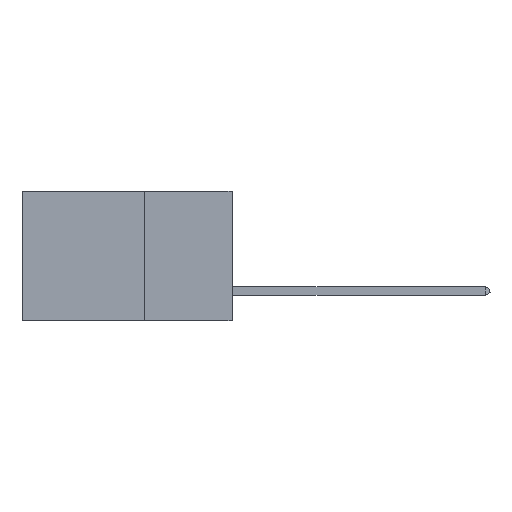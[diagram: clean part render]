
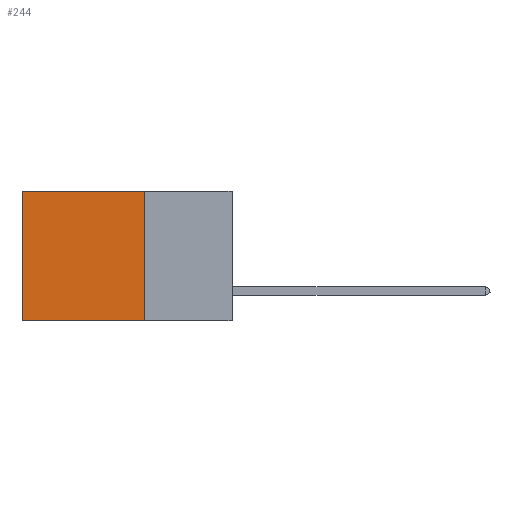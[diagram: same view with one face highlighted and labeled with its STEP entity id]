
A CAD part, left-side view. The second image highlights one B-rep face of the part: STEP entity #244.
In plain terms, the highlighted planar face has unit normal (-1, 0, 0).
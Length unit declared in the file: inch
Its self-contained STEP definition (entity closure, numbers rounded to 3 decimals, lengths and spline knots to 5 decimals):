
#244 = ADVANCED_FACE ( 'NONE', ( #23558 ), #25491, .F. ) ;
#1294 = CARTESIAN_POINT ( 'NONE',  ( 0.2875, 0.25, -0.37 ) ) ;
#1645 = CARTESIAN_POINT ( 'NONE',  ( 0.2875, 0.6, 0. ) ) ;
#3021 = DIRECTION ( 'NONE',  ( 1., 0., 0. ) ) ;
#3877 = DIRECTION ( 'NONE',  ( 0., 1., 0. ) ) ;
#4252 = DIRECTION ( 'NONE',  ( 0., 0., -1. ) ) ;
#5170 = VERTEX_POINT ( 'NONE', #14867 ) ;
#5262 = ORIENTED_EDGE ( 'NONE', *, *, #14628, .F. ) ;
#5477 = VERTEX_POINT ( 'NONE', #32260 ) ;
#5738 = DIRECTION ( 'NONE',  ( 0., 0., -1. ) ) ;
#6174 = LINE ( 'NONE', #23810, #12834 ) ;
#7422 = DIRECTION ( 'NONE',  ( 0., 0., -1. ) ) ;
#8686 = EDGE_CURVE ( 'NONE', #5170, #5477, #6174, .T. ) ;
#10539 = CARTESIAN_POINT ( 'NONE',  ( 0.2875, 0.6, -0.37 ) ) ;
#11924 = VECTOR ( 'NONE', #3877, 39.37008 ) ;
#12834 = VECTOR ( 'NONE', #31537, 39.37008 ) ;
#13616 = CARTESIAN_POINT ( 'NONE',  ( 0.2875, 0.25, 0. ) ) ;
#14628 = EDGE_CURVE ( 'NONE', #24508, #17805, #31287, .T. ) ;
#14867 = CARTESIAN_POINT ( 'NONE',  ( 0.2875, 0.25, 0. ) ) ;
#15395 = EDGE_CURVE ( 'NONE', #5477, #17805, #20969, .T. ) ;
#17216 = CARTESIAN_POINT ( 'NONE',  ( 0.2875, 0.25, -0.37 ) ) ;
#17805 = VERTEX_POINT ( 'NONE', #10539 ) ;
#20969 = LINE ( 'NONE', #1645, #30138 ) ;
#23020 = VECTOR ( 'NONE', #7422, 39.37008 ) ;
#23353 = EDGE_CURVE ( 'NONE', #5170, #24508, #29758, .T. ) ;
#23558 = FACE_OUTER_BOUND ( 'NONE', #28272, .T. ) ;
#23810 = CARTESIAN_POINT ( 'NONE',  ( 0.2875, 0.25, 0. ) ) ;
#23942 = ORIENTED_EDGE ( 'NONE', *, *, #15395, .T. ) ;
#24248 = ORIENTED_EDGE ( 'NONE', *, *, #23353, .F. ) ;
#24508 = VERTEX_POINT ( 'NONE', #17216 ) ;
#25491 = PLANE ( 'NONE',  #28406 ) ;
#27929 = ORIENTED_EDGE ( 'NONE', *, *, #8686, .T. ) ;
#28058 = CARTESIAN_POINT ( 'NONE',  ( 0.2875, 0.25, 0. ) ) ;
#28272 = EDGE_LOOP ( 'NONE', ( #23942, #5262, #24248, #27929 ) ) ;
#28406 = AXIS2_PLACEMENT_3D ( 'NONE', #28058, #3021, #5738 ) ;
#29758 = LINE ( 'NONE', #13616, #23020 ) ;
#30138 = VECTOR ( 'NONE', #4252, 39.37008 ) ;
#31287 = LINE ( 'NONE', #1294, #11924 ) ;
#31537 = DIRECTION ( 'NONE',  ( 0., 1., 0. ) ) ;
#32260 = CARTESIAN_POINT ( 'NONE',  ( 0.2875, 0.6, 0. ) ) ;
